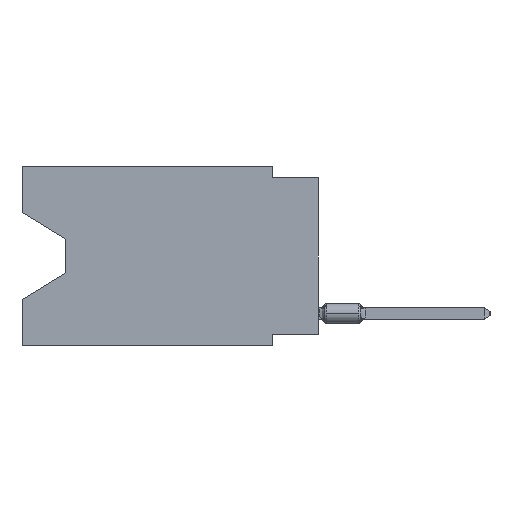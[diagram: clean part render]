
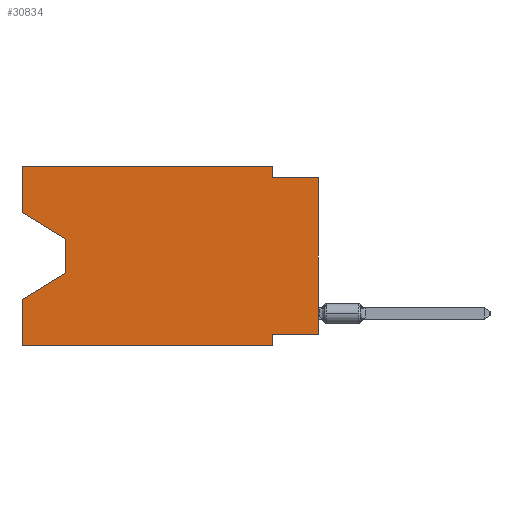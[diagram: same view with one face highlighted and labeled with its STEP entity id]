
A CAD part, left-side view. The second image highlights one B-rep face of the part: STEP entity #30834.
In plain terms, the highlighted planar face has unit normal (-1, 0, 0).
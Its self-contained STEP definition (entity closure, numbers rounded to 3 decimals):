
#234 = DIRECTION ( 'NONE',  ( 0., 0., 1. ) ) ;
#378 = VECTOR ( 'NONE', #10144, 1000. ) ;
#1229 = VECTOR ( 'NONE', #6345, 1000. ) ;
#1357 = DIRECTION ( 'NONE',  ( 0., 0., 1. ) ) ;
#1422 = CARTESIAN_POINT ( 'NONE',  ( 0., 2.54, 0. ) ) ;
#1841 = VECTOR ( 'NONE', #37312, 1000. ) ;
#2603 = AXIS2_PLACEMENT_3D ( 'NONE', #38967, #39869, #17945 ) ;
#2692 = VECTOR ( 'NONE', #34996, 1000. ) ;
#2832 = ORIENTED_EDGE ( 'NONE', *, *, #36202, .T. ) ;
#3395 = CARTESIAN_POINT ( 'NONE',  ( 0., 13.97, -5.893 ) ) ;
#4463 = EDGE_CURVE ( 'NONE', #18002, #20129, #5978, .T. ) ;
#5081 = VERTEX_POINT ( 'NONE', #44959 ) ;
#5691 = ORIENTED_EDGE ( 'NONE', *, *, #33778, .F. ) ;
#5978 = LINE ( 'NONE', #33057, #19950 ) ;
#6345 = DIRECTION ( 'NONE',  ( 0., 0., -1. ) ) ;
#6446 = ORIENTED_EDGE ( 'NONE', *, *, #36408, .T. ) ;
#7203 = CARTESIAN_POINT ( 'NONE',  ( 0., 16.383, 0. ) ) ;
#7227 = ORIENTED_EDGE ( 'NONE', *, *, #29145, .F. ) ;
#7744 = ORIENTED_EDGE ( 'NONE', *, *, #16779, .T. ) ;
#7991 = LINE ( 'NONE', #15160, #1841 ) ;
#8509 = DIRECTION ( 'NONE',  ( 0., -1., 0. ) ) ;
#10068 = VECTOR ( 'NONE', #234, 1000. ) ;
#10144 = DIRECTION ( 'NONE',  ( 0., -1., 0. ) ) ;
#10784 = DIRECTION ( 'NONE',  ( 0., 0., 1. ) ) ;
#10796 = PLANE ( 'NONE',  #2603 ) ;
#10960 = CARTESIAN_POINT ( 'NONE',  ( 0., 16.383, -9.906 ) ) ;
#11298 = ORIENTED_EDGE ( 'NONE', *, *, #34372, .T. ) ;
#11662 = CARTESIAN_POINT ( 'NONE',  ( 0., 0., -0.635 ) ) ;
#11752 = ORIENTED_EDGE ( 'NONE', *, *, #19286, .F. ) ;
#12770 = EDGE_LOOP ( 'NONE', ( #11298, #6446, #18992, #5691, #7744, #11752, #19180, #2832, #19237, #44309, #7227, #42732 ) ) ;
#12891 = CARTESIAN_POINT ( 'NONE',  ( 0., 16.383, -2.546 ) ) ;
#14366 = LINE ( 'NONE', #7203, #10068 ) ;
#14583 = EDGE_CURVE ( 'NONE', #32106, #26326, #7991, .T. ) ;
#15160 = CARTESIAN_POINT ( 'NONE',  ( 0., 0., -9.271 ) ) ;
#15348 = CARTESIAN_POINT ( 'NONE',  ( 0., 2.54, -9.906 ) ) ;
#16779 = EDGE_CURVE ( 'NONE', #42952, #18431, #37873, .T. ) ;
#17853 = VERTEX_POINT ( 'NONE', #3395 ) ;
#17945 = DIRECTION ( 'NONE',  ( 0., 0., -1. ) ) ;
#18002 = VERTEX_POINT ( 'NONE', #43551 ) ;
#18431 = VERTEX_POINT ( 'NONE', #15348 ) ;
#18992 = ORIENTED_EDGE ( 'NONE', *, *, #29311, .T. ) ;
#19180 = ORIENTED_EDGE ( 'NONE', *, *, #14583, .F. ) ;
#19237 = ORIENTED_EDGE ( 'NONE', *, *, #19634, .F. ) ;
#19286 = EDGE_CURVE ( 'NONE', #26326, #18431, #37331, .T. ) ;
#19634 = EDGE_CURVE ( 'NONE', #37476, #43106, #36149, .T. ) ;
#19950 = VECTOR ( 'NONE', #1357, 1000. ) ;
#20129 = VERTEX_POINT ( 'NONE', #21549 ) ;
#20620 = CARTESIAN_POINT ( 'NONE',  ( 0., 13.97, -4.013 ) ) ;
#21103 = VECTOR ( 'NONE', #8509, 1000. ) ;
#21210 = VECTOR ( 'NONE', #33666, 1000. ) ;
#21549 = CARTESIAN_POINT ( 'NONE',  ( 0., 16.383, 0. ) ) ;
#21797 = EDGE_CURVE ( 'NONE', #31091, #37476, #32150, .T. ) ;
#22187 = DIRECTION ( 'NONE',  ( 0., 0., -1. ) ) ;
#22423 = CARTESIAN_POINT ( 'NONE',  ( 0., 2.54, 0. ) ) ;
#23693 = CARTESIAN_POINT ( 'NONE',  ( 0., 2.54, -9.906 ) ) ;
#24143 = CARTESIAN_POINT ( 'NONE',  ( 0., 2.54, -9.271 ) ) ;
#25657 = VECTOR ( 'NONE', #39385, 1000. ) ;
#26326 = VERTEX_POINT ( 'NONE', #24143 ) ;
#28641 = VECTOR ( 'NONE', #10784, 1000. ) ;
#29023 = LINE ( 'NONE', #35281, #28641 ) ;
#29145 = EDGE_CURVE ( 'NONE', #20129, #31091, #36689, .T. ) ;
#29263 = FACE_OUTER_BOUND ( 'NONE', #12770, .T. ) ;
#29311 = EDGE_CURVE ( 'NONE', #17853, #5081, #37822, .T. ) ;
#30435 = LINE ( 'NONE', #12891, #2692 ) ;
#30834 = ADVANCED_FACE ( 'NONE', ( #29263 ), #10796, .F. ) ;
#31091 = VERTEX_POINT ( 'NONE', #1422 ) ;
#32106 = VERTEX_POINT ( 'NONE', #38888 ) ;
#32150 = LINE ( 'NONE', #22423, #32557 ) ;
#32557 = VECTOR ( 'NONE', #22187, 1000. ) ;
#33057 = CARTESIAN_POINT ( 'NONE',  ( 0., 16.383, 0. ) ) ;
#33666 = DIRECTION ( 'NONE',  ( 0., 0., -1. ) ) ;
#33704 = CARTESIAN_POINT ( 'NONE',  ( 0., 16.383, 0. ) ) ;
#33778 = EDGE_CURVE ( 'NONE', #42952, #5081, #14366, .T. ) ;
#33885 = CARTESIAN_POINT ( 'NONE',  ( 0., 2.54, -0.635 ) ) ;
#34157 = CARTESIAN_POINT ( 'NONE',  ( 0., 13.97, -5.893 ) ) ;
#34372 = EDGE_CURVE ( 'NONE', #18002, #41640, #30435, .T. ) ;
#34996 = DIRECTION ( 'NONE',  ( 0., -0.855, -0.519 ) ) ;
#35281 = CARTESIAN_POINT ( 'NONE',  ( 0., 0., 0. ) ) ;
#36149 = LINE ( 'NONE', #11662, #25657 ) ;
#36202 = EDGE_CURVE ( 'NONE', #32106, #43106, #29023, .T. ) ;
#36408 = EDGE_CURVE ( 'NONE', #41640, #17853, #40985, .T. ) ;
#36689 = LINE ( 'NONE', #33704, #21103 ) ;
#37312 = DIRECTION ( 'NONE',  ( 0., 1., 0. ) ) ;
#37314 = CARTESIAN_POINT ( 'NONE',  ( 0., 0., -0.635 ) ) ;
#37331 = LINE ( 'NONE', #23693, #21210 ) ;
#37476 = VERTEX_POINT ( 'NONE', #33885 ) ;
#37822 = LINE ( 'NONE', #34157, #43238 ) ;
#37873 = LINE ( 'NONE', #41765, #378 ) ;
#38888 = CARTESIAN_POINT ( 'NONE',  ( 0., 0., -9.271 ) ) ;
#38967 = CARTESIAN_POINT ( 'NONE',  ( 0., 16.383, 0. ) ) ;
#39385 = DIRECTION ( 'NONE',  ( 0., -1., 0. ) ) ;
#39869 = DIRECTION ( 'NONE',  ( 1., 0., 0. ) ) ;
#40985 = LINE ( 'NONE', #44662, #1229 ) ;
#41640 = VERTEX_POINT ( 'NONE', #20620 ) ;
#41717 = DIRECTION ( 'NONE',  ( 0., 0.855, -0.519 ) ) ;
#41765 = CARTESIAN_POINT ( 'NONE',  ( 0., 16.383, -9.906 ) ) ;
#42732 = ORIENTED_EDGE ( 'NONE', *, *, #4463, .F. ) ;
#42952 = VERTEX_POINT ( 'NONE', #10960 ) ;
#43106 = VERTEX_POINT ( 'NONE', #37314 ) ;
#43238 = VECTOR ( 'NONE', #41717, 1000. ) ;
#43551 = CARTESIAN_POINT ( 'NONE',  ( 0., 16.383, -2.546 ) ) ;
#44309 = ORIENTED_EDGE ( 'NONE', *, *, #21797, .F. ) ;
#44662 = CARTESIAN_POINT ( 'NONE',  ( 0., 13.97, -4.013 ) ) ;
#44959 = CARTESIAN_POINT ( 'NONE',  ( 0., 16.383, -7.36 ) ) ;
